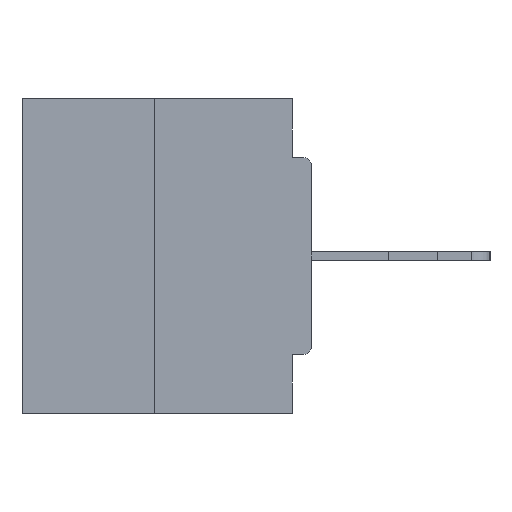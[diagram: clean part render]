
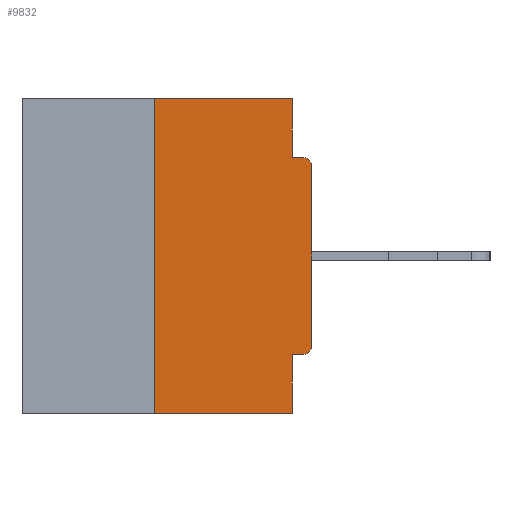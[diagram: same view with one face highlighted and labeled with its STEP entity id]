
A CAD part, left-side view. The second image highlights one B-rep face of the part: STEP entity #9832.
In plain terms, the highlighted planar face has unit normal (-1, 0, 0).
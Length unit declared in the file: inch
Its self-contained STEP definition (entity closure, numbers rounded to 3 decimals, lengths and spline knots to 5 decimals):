
#497 = CARTESIAN_POINT ( 'NONE',  ( 0., 0.031, -0.5 ) ) ;
#742 = CARTESIAN_POINT ( 'NONE',  ( 0., 0., -0.3915 ) ) ;
#870 = DIRECTION ( 'NONE',  ( 0., 0., 1. ) ) ;
#1321 = CARTESIAN_POINT ( 'NONE',  ( 0., 0., 0. ) ) ;
#1555 = DIRECTION ( 'NONE',  ( 0., 0., 1. ) ) ;
#2845 = EDGE_CURVE ( 'NONE', #16591, #17806, #18420, .T. ) ;
#3078 = CARTESIAN_POINT ( 'NONE',  ( 0., 0.031, -0.0935 ) ) ;
#3147 = EDGE_CURVE ( 'NONE', #5370, #26169, #27458, .T. ) ;
#3829 = ORIENTED_EDGE ( 'NONE', *, *, #6802, .F. ) ;
#3896 = VERTEX_POINT ( 'NONE', #7305 ) ;
#3928 = DIRECTION ( 'NONE',  ( 0., 0., -1. ) ) ;
#5370 = VERTEX_POINT ( 'NONE', #742 ) ;
#5995 = DIRECTION ( 'NONE',  ( -1., 0., 0. ) ) ;
#6056 = VECTOR ( 'NONE', #6183, 39.37008 ) ;
#6183 = DIRECTION ( 'NONE',  ( 0., 1., 0. ) ) ;
#6564 = PLANE ( 'NONE',  #26273 ) ;
#6802 = EDGE_CURVE ( 'NONE', #3896, #26327, #17795, .T. ) ;
#6854 = EDGE_CURVE ( 'NONE', #17710, #16591, #25305, .T. ) ;
#7305 = CARTESIAN_POINT ( 'NONE',  ( 0., 0.015, -0.4065 ) ) ;
#7553 = EDGE_CURVE ( 'NONE', #28026, #17710, #22582, .T. ) ;
#7669 = EDGE_CURVE ( 'NONE', #27612, #28063, #27714, .T. ) ;
#7709 = ORIENTED_EDGE ( 'NONE', *, *, #7553, .F. ) ;
#8429 = CIRCLE ( 'NONE', #12434, 0.015 ) ;
#9832 = ADVANCED_FACE ( 'NONE', ( #16614 ), #6564, .F. ) ;
#10030 = DIRECTION ( 'NONE',  ( 0., -1., 0. ) ) ;
#11509 = CARTESIAN_POINT ( 'NONE',  ( 0., 0., -0.0935 ) ) ;
#12249 = DIRECTION ( 'NONE',  ( 0., 0., -1. ) ) ;
#12396 = CARTESIAN_POINT ( 'NONE',  ( 0., 0.46, 0. ) ) ;
#12434 = AXIS2_PLACEMENT_3D ( 'NONE', #18377, #5995, #20553 ) ;
#13153 = DIRECTION ( 'NONE',  ( 0., -1., 0. ) ) ;
#13715 = EDGE_CURVE ( 'NONE', #26327, #28063, #15906, .T. ) ;
#13760 = LINE ( 'NONE', #23023, #17342 ) ;
#15901 = DIRECTION ( 'NONE',  ( 0., 0., -1. ) ) ;
#15906 = LINE ( 'NONE', #25611, #20339 ) ;
#16056 = DIRECTION ( 'NONE',  ( 0., 0., -1. ) ) ;
#16591 = VERTEX_POINT ( 'NONE', #3078 ) ;
#16614 = FACE_OUTER_BOUND ( 'NONE', #22853, .T. ) ;
#16631 = VECTOR ( 'NONE', #13153, 39.37008 ) ;
#16807 = ORIENTED_EDGE ( 'NONE', *, *, #21988, .T. ) ;
#16868 = CARTESIAN_POINT ( 'NONE',  ( 0., 0.25, -0.5 ) ) ;
#17342 = VECTOR ( 'NONE', #1555, 39.37008 ) ;
#17710 = VERTEX_POINT ( 'NONE', #24358 ) ;
#17795 = LINE ( 'NONE', #22803, #6056 ) ;
#17806 = VERTEX_POINT ( 'NONE', #29501 ) ;
#18377 = CARTESIAN_POINT ( 'NONE',  ( 0., 0.015, -0.3915 ) ) ;
#18420 = LINE ( 'NONE', #11509, #25161 ) ;
#18650 = CARTESIAN_POINT ( 'NONE',  ( 0., 0.46, 0. ) ) ;
#19025 = CARTESIAN_POINT ( 'NONE',  ( 0., 0., -0.1085 ) ) ;
#19149 = CARTESIAN_POINT ( 'NONE',  ( 0., 0.25, 0. ) ) ;
#19156 = CARTESIAN_POINT ( 'NONE',  ( 0., 0.015, -0.1085 ) ) ;
#19573 = VECTOR ( 'NONE', #15901, 39.37008 ) ;
#20099 = EDGE_CURVE ( 'NONE', #27612, #28026, #13760, .T. ) ;
#20339 = VECTOR ( 'NONE', #16056, 39.37008 ) ;
#20553 = DIRECTION ( 'NONE',  ( 0., 0., -1. ) ) ;
#21077 = DIRECTION ( 'NONE',  ( 0., -1., 0. ) ) ;
#21408 = ORIENTED_EDGE ( 'NONE', *, *, #20099, .F. ) ;
#21988 = EDGE_CURVE ( 'NONE', #3896, #5370, #8429, .T. ) ;
#22035 = CIRCLE ( 'NONE', #30476, 0.015 ) ;
#22133 = VECTOR ( 'NONE', #10030, 39.37008 ) ;
#22175 = ORIENTED_EDGE ( 'NONE', *, *, #23322, .T. ) ;
#22224 = ORIENTED_EDGE ( 'NONE', *, *, #13715, .F. ) ;
#22582 = LINE ( 'NONE', #12396, #22133 ) ;
#22803 = CARTESIAN_POINT ( 'NONE',  ( 0., 0., -0.4065 ) ) ;
#22853 = EDGE_LOOP ( 'NONE', ( #7709, #21408, #27316, #22224, #3829, #16807, #30303, #22175, #29326, #26441 ) ) ;
#23023 = CARTESIAN_POINT ( 'NONE',  ( 0., 0.25, 0. ) ) ;
#23322 = EDGE_CURVE ( 'NONE', #26169, #17806, #22035, .T. ) ;
#24358 = CARTESIAN_POINT ( 'NONE',  ( 0., 0.031, 0. ) ) ;
#24955 = VECTOR ( 'NONE', #870, 39.37008 ) ;
#25161 = VECTOR ( 'NONE', #21077, 39.37008 ) ;
#25305 = LINE ( 'NONE', #27938, #19573 ) ;
#25611 = CARTESIAN_POINT ( 'NONE',  ( 0., 0.031, -0.5 ) ) ;
#26169 = VERTEX_POINT ( 'NONE', #19025 ) ;
#26208 = DIRECTION ( 'NONE',  ( -1., 0., 0. ) ) ;
#26273 = AXIS2_PLACEMENT_3D ( 'NONE', #18650, #30512, #3928 ) ;
#26327 = VERTEX_POINT ( 'NONE', #26530 ) ;
#26441 = ORIENTED_EDGE ( 'NONE', *, *, #6854, .F. ) ;
#26530 = CARTESIAN_POINT ( 'NONE',  ( 0., 0.031, -0.4065 ) ) ;
#27316 = ORIENTED_EDGE ( 'NONE', *, *, #7669, .T. ) ;
#27458 = LINE ( 'NONE', #1321, #24955 ) ;
#27612 = VERTEX_POINT ( 'NONE', #16868 ) ;
#27714 = LINE ( 'NONE', #30197, #16631 ) ;
#27938 = CARTESIAN_POINT ( 'NONE',  ( 0., 0.031, 0. ) ) ;
#28026 = VERTEX_POINT ( 'NONE', #19149 ) ;
#28063 = VERTEX_POINT ( 'NONE', #497 ) ;
#29326 = ORIENTED_EDGE ( 'NONE', *, *, #2845, .F. ) ;
#29501 = CARTESIAN_POINT ( 'NONE',  ( 0., 0.015, -0.0935 ) ) ;
#30197 = CARTESIAN_POINT ( 'NONE',  ( 0., 0.46, -0.5 ) ) ;
#30303 = ORIENTED_EDGE ( 'NONE', *, *, #3147, .T. ) ;
#30476 = AXIS2_PLACEMENT_3D ( 'NONE', #19156, #26208, #12249 ) ;
#30512 = DIRECTION ( 'NONE',  ( 1., 0., 0. ) ) ;
